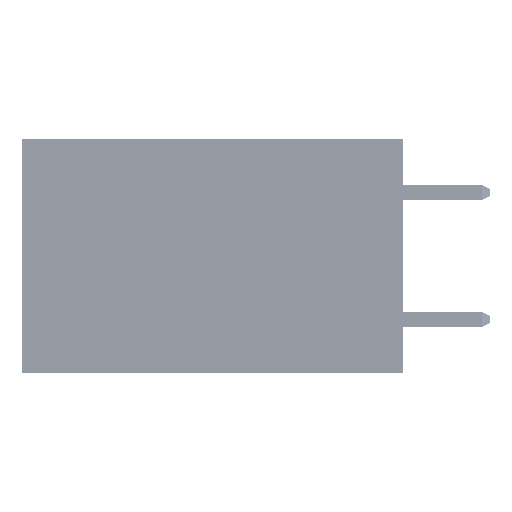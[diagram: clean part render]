
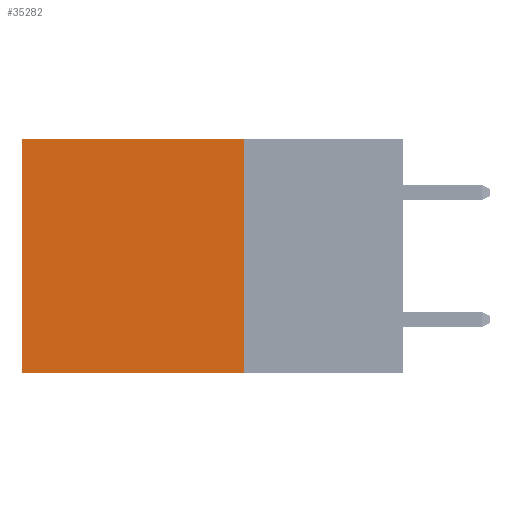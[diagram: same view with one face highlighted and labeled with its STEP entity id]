
A CAD part, left-side view. The second image highlights one B-rep face of the part: STEP entity #35282.
In plain terms, the highlighted planar face has unit normal (-1, 0, 0).
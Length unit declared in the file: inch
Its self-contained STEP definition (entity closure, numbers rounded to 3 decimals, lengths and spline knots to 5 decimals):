
#1866 = VECTOR ( 'NONE', #44205, 39.37008 ) ;
#6127 = CARTESIAN_POINT ( 'NONE',  ( 0.2875, 0.25, 0. ) ) ;
#6606 = EDGE_CURVE ( 'NONE', #22995, #38874, #36856, .T. ) ;
#7106 = AXIS2_PLACEMENT_3D ( 'NONE', #6127, #14117, #42806 ) ;
#10253 = CARTESIAN_POINT ( 'NONE',  ( 0.2875, 0.25, 0. ) ) ;
#13043 = DIRECTION ( 'NONE',  ( 0., 0., -1. ) ) ;
#13150 = EDGE_CURVE ( 'NONE', #26524, #33871, #37480, .T. ) ;
#13304 = EDGE_CURVE ( 'NONE', #22995, #26524, #23679, .T. ) ;
#14117 = DIRECTION ( 'NONE',  ( 1., 0., 0. ) ) ;
#14698 = ORIENTED_EDGE ( 'NONE', *, *, #23760, .T. ) ;
#19812 = ORIENTED_EDGE ( 'NONE', *, *, #6606, .T. ) ;
#21564 = CARTESIAN_POINT ( 'NONE',  ( 0.2875, 0.25, 0. ) ) ;
#22777 = CARTESIAN_POINT ( 'NONE',  ( 0.2875, 0.6, -0.37 ) ) ;
#22995 = VERTEX_POINT ( 'NONE', #10253 ) ;
#23065 = VECTOR ( 'NONE', #13043, 39.37008 ) ;
#23679 = LINE ( 'NONE', #40655, #23065 ) ;
#23760 = EDGE_CURVE ( 'NONE', #38874, #33871, #29210, .T. ) ;
#26524 = VERTEX_POINT ( 'NONE', #28487 ) ;
#27750 = ORIENTED_EDGE ( 'NONE', *, *, #13304, .F. ) ;
#28487 = CARTESIAN_POINT ( 'NONE',  ( 0.2875, 0.25, -0.37 ) ) ;
#29210 = LINE ( 'NONE', #50585, #29813 ) ;
#29813 = VECTOR ( 'NONE', #42892, 39.37008 ) ;
#30194 = PLANE ( 'NONE',  #7106 ) ;
#30293 = DIRECTION ( 'NONE',  ( 0., 1., 0. ) ) ;
#33871 = VERTEX_POINT ( 'NONE', #22777 ) ;
#35282 = ADVANCED_FACE ( 'NONE', ( #42219 ), #30194, .F. ) ;
#36186 = ORIENTED_EDGE ( 'NONE', *, *, #13150, .F. ) ;
#36856 = LINE ( 'NONE', #21564, #43149 ) ;
#37480 = LINE ( 'NONE', #47697, #1866 ) ;
#38874 = VERTEX_POINT ( 'NONE', #39322 ) ;
#39322 = CARTESIAN_POINT ( 'NONE',  ( 0.2875, 0.6, 0. ) ) ;
#40655 = CARTESIAN_POINT ( 'NONE',  ( 0.2875, 0.25, 0. ) ) ;
#42219 = FACE_OUTER_BOUND ( 'NONE', #45051, .T. ) ;
#42806 = DIRECTION ( 'NONE',  ( 0., 0., -1. ) ) ;
#42892 = DIRECTION ( 'NONE',  ( 0., 0., -1. ) ) ;
#43149 = VECTOR ( 'NONE', #30293, 39.37008 ) ;
#44205 = DIRECTION ( 'NONE',  ( 0., 1., 0. ) ) ;
#45051 = EDGE_LOOP ( 'NONE', ( #14698, #36186, #27750, #19812 ) ) ;
#47697 = CARTESIAN_POINT ( 'NONE',  ( 0.2875, 0.25, -0.37 ) ) ;
#50585 = CARTESIAN_POINT ( 'NONE',  ( 0.2875, 0.6, 0. ) ) ;
